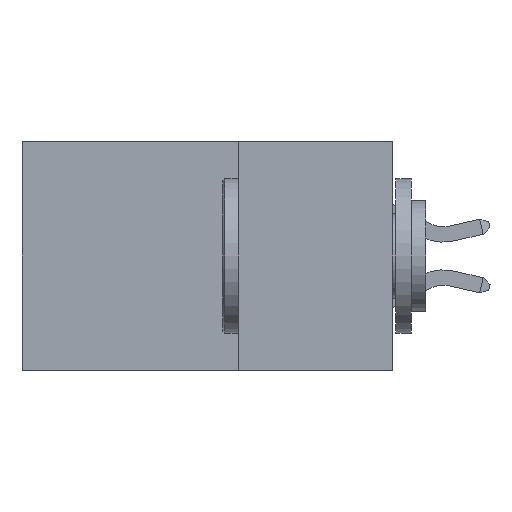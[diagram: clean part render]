
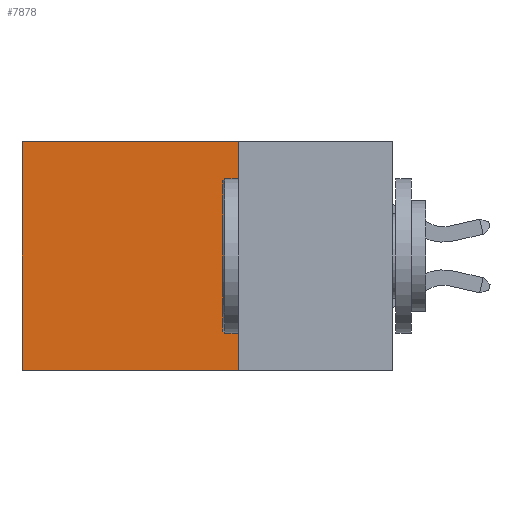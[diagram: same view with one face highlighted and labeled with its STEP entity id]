
A CAD part, left-side view. The second image highlights one B-rep face of the part: STEP entity #7878.
In plain terms, the highlighted planar face has unit normal (-1, 0, 0).
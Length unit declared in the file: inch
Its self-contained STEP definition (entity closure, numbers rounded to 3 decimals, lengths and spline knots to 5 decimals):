
#17 = CARTESIAN_POINT ( 'NONE',  ( 0.2875, 0.6, 0. ) ) ;
#211 = EDGE_CURVE ( 'NONE', #6458, #17609, #1485, .T. ) ;
#381 = DIRECTION ( 'NONE',  ( 0., 1., 0. ) ) ;
#969 = PLANE ( 'NONE',  #15600 ) ;
#1485 = LINE ( 'NONE', #20649, #22773 ) ;
#2996 = ORIENTED_EDGE ( 'NONE', *, *, #4529, .F. ) ;
#3597 = EDGE_CURVE ( 'NONE', #9871, #6458, #10642, .T. ) ;
#3645 = EDGE_CURVE ( 'NONE', #9871, #6418, #20700, .T. ) ;
#4529 = EDGE_CURVE ( 'NONE', #6418, #17609, #5760, .T. ) ;
#4734 = ORIENTED_EDGE ( 'NONE', *, *, #3645, .F. ) ;
#5760 = LINE ( 'NONE', #6419, #6742 ) ;
#6084 = DIRECTION ( 'NONE',  ( 0., 0., -1. ) ) ;
#6418 = VERTEX_POINT ( 'NONE', #16532 ) ;
#6419 = CARTESIAN_POINT ( 'NONE',  ( 0.2875, 0.25, -0.37 ) ) ;
#6458 = VERTEX_POINT ( 'NONE', #17 ) ;
#6742 = VECTOR ( 'NONE', #8568, 39.37008 ) ;
#7288 = FACE_OUTER_BOUND ( 'NONE', #8153, .T. ) ;
#7878 = ADVANCED_FACE ( 'NONE', ( #7288 ), #969, .F. ) ;
#8153 = EDGE_LOOP ( 'NONE', ( #12303, #2996, #4734, #13173 ) ) ;
#8568 = DIRECTION ( 'NONE',  ( 0., 1., 0. ) ) ;
#9390 = DIRECTION ( 'NONE',  ( 1., 0., 0. ) ) ;
#9871 = VERTEX_POINT ( 'NONE', #11010 ) ;
#10230 = DIRECTION ( 'NONE',  ( 0., 0., -1. ) ) ;
#10642 = LINE ( 'NONE', #26308, #11290 ) ;
#11010 = CARTESIAN_POINT ( 'NONE',  ( 0.2875, 0.25, 0. ) ) ;
#11290 = VECTOR ( 'NONE', #381, 39.37008 ) ;
#12303 = ORIENTED_EDGE ( 'NONE', *, *, #211, .T. ) ;
#13173 = ORIENTED_EDGE ( 'NONE', *, *, #3597, .T. ) ;
#13223 = CARTESIAN_POINT ( 'NONE',  ( 0.2875, 0.6, -0.37 ) ) ;
#15600 = AXIS2_PLACEMENT_3D ( 'NONE', #21795, #9390, #25837 ) ;
#16532 = CARTESIAN_POINT ( 'NONE',  ( 0.2875, 0.25, -0.37 ) ) ;
#17609 = VERTEX_POINT ( 'NONE', #13223 ) ;
#20649 = CARTESIAN_POINT ( 'NONE',  ( 0.2875, 0.6, 0. ) ) ;
#20700 = LINE ( 'NONE', #22622, #26491 ) ;
#21795 = CARTESIAN_POINT ( 'NONE',  ( 0.2875, 0.25, 0. ) ) ;
#22622 = CARTESIAN_POINT ( 'NONE',  ( 0.2875, 0.25, 0. ) ) ;
#22773 = VECTOR ( 'NONE', #6084, 39.37008 ) ;
#25837 = DIRECTION ( 'NONE',  ( 0., 0., -1. ) ) ;
#26308 = CARTESIAN_POINT ( 'NONE',  ( 0.2875, 0.25, 0. ) ) ;
#26491 = VECTOR ( 'NONE', #10230, 39.37008 ) ;
